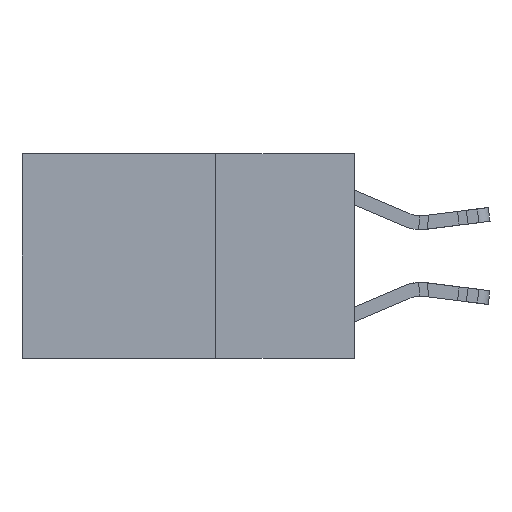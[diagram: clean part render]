
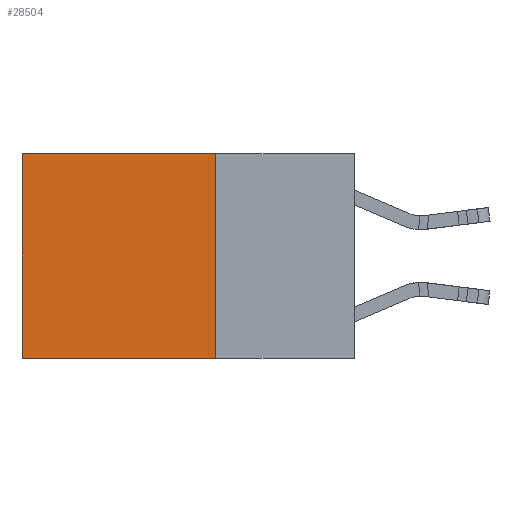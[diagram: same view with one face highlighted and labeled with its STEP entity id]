
A CAD part, left-side view. The second image highlights one B-rep face of the part: STEP entity #28504.
In plain terms, the highlighted planar face has unit normal (-1, 0, 0).
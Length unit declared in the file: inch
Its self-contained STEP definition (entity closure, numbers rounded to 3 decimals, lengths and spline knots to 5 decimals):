
#854 = DIRECTION ( 'NONE',  ( 0., 1., 0. ) ) ;
#1926 = VERTEX_POINT ( 'NONE', #3433 ) ;
#3046 = VECTOR ( 'NONE', #17936, 39.37008 ) ;
#3387 = LINE ( 'NONE', #27463, #17347 ) ;
#3433 = CARTESIAN_POINT ( 'NONE',  ( 0.2625, 0.6, 0. ) ) ;
#3952 = ORIENTED_EDGE ( 'NONE', *, *, #27369, .T. ) ;
#4108 = FACE_OUTER_BOUND ( 'NONE', #27549, .T. ) ;
#7138 = EDGE_CURVE ( 'NONE', #8203, #18253, #22528, .T. ) ;
#8203 = VERTEX_POINT ( 'NONE', #11674 ) ;
#9084 = DIRECTION ( 'NONE',  ( 0., 1., 0. ) ) ;
#9180 = PLANE ( 'NONE',  #9512 ) ;
#9512 = AXIS2_PLACEMENT_3D ( 'NONE', #11738, #13806, #11106 ) ;
#10050 = EDGE_CURVE ( 'NONE', #18253, #13172, #11488, .T. ) ;
#11106 = DIRECTION ( 'NONE',  ( 0., 0., -1. ) ) ;
#11488 = LINE ( 'NONE', #21136, #19177 ) ;
#11674 = CARTESIAN_POINT ( 'NONE',  ( 0.2625, 0.25, 0. ) ) ;
#11738 = CARTESIAN_POINT ( 'NONE',  ( 0.2625, 0.25, 0. ) ) ;
#11751 = CARTESIAN_POINT ( 'NONE',  ( 0.2625, 0.6, -0.37 ) ) ;
#13172 = VERTEX_POINT ( 'NONE', #11751 ) ;
#13245 = LINE ( 'NONE', #22584, #14057 ) ;
#13806 = DIRECTION ( 'NONE',  ( 1., 0., 0. ) ) ;
#14057 = VECTOR ( 'NONE', #854, 39.37008 ) ;
#15560 = EDGE_CURVE ( 'NONE', #1926, #13172, #3387, .T. ) ;
#15729 = CARTESIAN_POINT ( 'NONE',  ( 0.2625, 0.25, 0. ) ) ;
#15868 = ORIENTED_EDGE ( 'NONE', *, *, #15560, .T. ) ;
#16883 = CARTESIAN_POINT ( 'NONE',  ( 0.2625, 0.25, -0.37 ) ) ;
#17347 = VECTOR ( 'NONE', #27304, 39.37008 ) ;
#17936 = DIRECTION ( 'NONE',  ( 0., 0., -1. ) ) ;
#18253 = VERTEX_POINT ( 'NONE', #16883 ) ;
#19177 = VECTOR ( 'NONE', #9084, 39.37008 ) ;
#21136 = CARTESIAN_POINT ( 'NONE',  ( 0.2625, 0.25, -0.37 ) ) ;
#21526 = ORIENTED_EDGE ( 'NONE', *, *, #10050, .F. ) ;
#22528 = LINE ( 'NONE', #15729, #3046 ) ;
#22584 = CARTESIAN_POINT ( 'NONE',  ( 0.2625, 0.25, 0. ) ) ;
#27304 = DIRECTION ( 'NONE',  ( 0., 0., -1. ) ) ;
#27369 = EDGE_CURVE ( 'NONE', #8203, #1926, #13245, .T. ) ;
#27463 = CARTESIAN_POINT ( 'NONE',  ( 0.2625, 0.6, 0. ) ) ;
#27549 = EDGE_LOOP ( 'NONE', ( #15868, #21526, #29272, #3952 ) ) ;
#28504 = ADVANCED_FACE ( 'NONE', ( #4108 ), #9180, .F. ) ;
#29272 = ORIENTED_EDGE ( 'NONE', *, *, #7138, .F. ) ;
